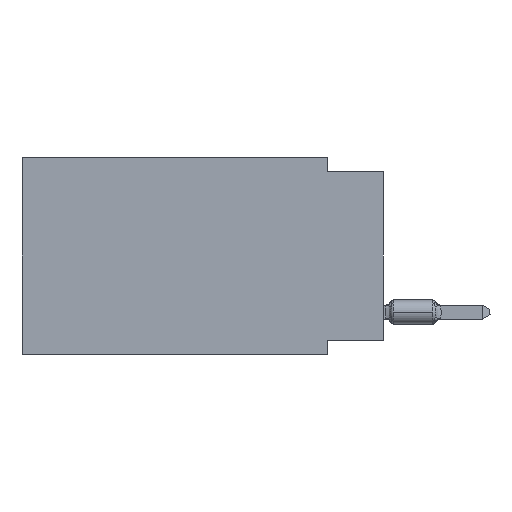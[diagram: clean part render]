
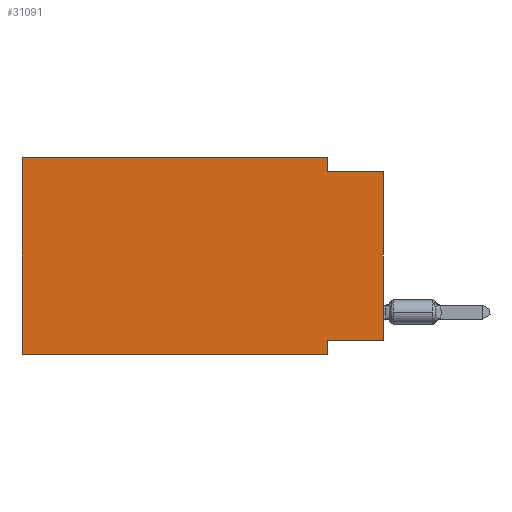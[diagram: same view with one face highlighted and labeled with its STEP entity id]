
A CAD part, left-side view. The second image highlights one B-rep face of the part: STEP entity #31091.
In plain terms, the highlighted planar face has unit normal (-1, 0, 0).
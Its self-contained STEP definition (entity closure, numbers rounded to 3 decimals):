
#676 = VECTOR ( 'NONE', #26741, 1000. ) ;
#1044 = LINE ( 'NONE', #28769, #676 ) ;
#1393 = CARTESIAN_POINT ( 'NONE',  ( 0., 16.383, 0. ) ) ;
#1686 = CARTESIAN_POINT ( 'NONE',  ( 0., 16.383, -8.89 ) ) ;
#1898 = DIRECTION ( 'NONE',  ( 0., 0., -1. ) ) ;
#2497 = VECTOR ( 'NONE', #14791, 1000. ) ;
#2644 = EDGE_CURVE ( 'NONE', #17734, #23725, #25073, .T. ) ;
#3044 = ORIENTED_EDGE ( 'NONE', *, *, #18412, .F. ) ;
#3313 = VERTEX_POINT ( 'NONE', #30371 ) ;
#4046 = ORIENTED_EDGE ( 'NONE', *, *, #2644, .F. ) ;
#4210 = LINE ( 'NONE', #1686, #9690 ) ;
#4249 = VERTEX_POINT ( 'NONE', #11958 ) ;
#4305 = ORIENTED_EDGE ( 'NONE', *, *, #30564, .F. ) ;
#4411 = PLANE ( 'NONE',  #13729 ) ;
#4477 = CARTESIAN_POINT ( 'NONE',  ( 0., 2.54, -8.255 ) ) ;
#4632 = EDGE_CURVE ( 'NONE', #14432, #17476, #32420, .T. ) ;
#4674 = CARTESIAN_POINT ( 'NONE',  ( 0., 2.54, -0.635 ) ) ;
#6158 = CARTESIAN_POINT ( 'NONE',  ( 0., 16.383, 0. ) ) ;
#6249 = VECTOR ( 'NONE', #14885, 1000. ) ;
#6535 = CARTESIAN_POINT ( 'NONE',  ( 0., 16.383, 0. ) ) ;
#6783 = EDGE_CURVE ( 'NONE', #3313, #19375, #8744, .T. ) ;
#6998 = LINE ( 'NONE', #30048, #30743 ) ;
#7349 = DIRECTION ( 'NONE',  ( 0., 0., 1. ) ) ;
#8744 = LINE ( 'NONE', #32408, #9843 ) ;
#9025 = VERTEX_POINT ( 'NONE', #4477 ) ;
#9569 = CARTESIAN_POINT ( 'NONE',  ( 0., 0., -0.635 ) ) ;
#9690 = VECTOR ( 'NONE', #32082, 1000. ) ;
#9843 = VECTOR ( 'NONE', #7349, 1000. ) ;
#9968 = CARTESIAN_POINT ( 'NONE',  ( 0., 2.54, 0. ) ) ;
#11938 = ORIENTED_EDGE ( 'NONE', *, *, #29791, .F. ) ;
#11958 = CARTESIAN_POINT ( 'NONE',  ( 0., 2.54, -8.89 ) ) ;
#12544 = DIRECTION ( 'NONE',  ( 0., 0., -1. ) ) ;
#12728 = ORIENTED_EDGE ( 'NONE', *, *, #4632, .F. ) ;
#12847 = EDGE_CURVE ( 'NONE', #14432, #4249, #4210, .T. ) ;
#12972 = VECTOR ( 'NONE', #14708, 1000. ) ;
#13729 = AXIS2_PLACEMENT_3D ( 'NONE', #1393, #14586, #1898 ) ;
#13777 = EDGE_CURVE ( 'NONE', #23725, #19375, #1044, .T. ) ;
#14094 = FACE_OUTER_BOUND ( 'NONE', #30546, .T. ) ;
#14432 = VERTEX_POINT ( 'NONE', #20504 ) ;
#14586 = DIRECTION ( 'NONE',  ( 1., 0., 0. ) ) ;
#14708 = DIRECTION ( 'NONE',  ( 0., -1., 0. ) ) ;
#14791 = DIRECTION ( 'NONE',  ( 0., 1., 0. ) ) ;
#14885 = DIRECTION ( 'NONE',  ( 0., 0., 1. ) ) ;
#14891 = CARTESIAN_POINT ( 'NONE',  ( 0., 2.54, 0. ) ) ;
#17476 = VERTEX_POINT ( 'NONE', #6158 ) ;
#17734 = VERTEX_POINT ( 'NONE', #9968 ) ;
#18412 = EDGE_CURVE ( 'NONE', #17476, #17734, #19736, .T. ) ;
#19130 = ORIENTED_EDGE ( 'NONE', *, *, #6783, .T. ) ;
#19375 = VERTEX_POINT ( 'NONE', #9569 ) ;
#19736 = LINE ( 'NONE', #6535, #12972 ) ;
#19961 = LINE ( 'NONE', #24483, #2497 ) ;
#20504 = CARTESIAN_POINT ( 'NONE',  ( 0., 16.383, -8.89 ) ) ;
#23725 = VERTEX_POINT ( 'NONE', #4674 ) ;
#24483 = CARTESIAN_POINT ( 'NONE',  ( 0., 0., -8.255 ) ) ;
#24695 = DIRECTION ( 'NONE',  ( 0., 0., -1. ) ) ;
#25073 = LINE ( 'NONE', #14891, #28007 ) ;
#26741 = DIRECTION ( 'NONE',  ( 0., -1., 0. ) ) ;
#27108 = ORIENTED_EDGE ( 'NONE', *, *, #12847, .T. ) ;
#27401 = CARTESIAN_POINT ( 'NONE',  ( 0., 16.383, 0. ) ) ;
#28007 = VECTOR ( 'NONE', #12544, 1000. ) ;
#28404 = ORIENTED_EDGE ( 'NONE', *, *, #13777, .F. ) ;
#28769 = CARTESIAN_POINT ( 'NONE',  ( 0., 0., -0.635 ) ) ;
#29791 = EDGE_CURVE ( 'NONE', #9025, #4249, #6998, .T. ) ;
#30048 = CARTESIAN_POINT ( 'NONE',  ( 0., 2.54, -8.89 ) ) ;
#30371 = CARTESIAN_POINT ( 'NONE',  ( 0., 0., -8.255 ) ) ;
#30546 = EDGE_LOOP ( 'NONE', ( #19130, #28404, #4046, #3044, #12728, #27108, #11938, #4305 ) ) ;
#30564 = EDGE_CURVE ( 'NONE', #3313, #9025, #19961, .T. ) ;
#30743 = VECTOR ( 'NONE', #24695, 1000. ) ;
#31091 = ADVANCED_FACE ( 'NONE', ( #14094 ), #4411, .F. ) ;
#32082 = DIRECTION ( 'NONE',  ( 0., -1., 0. ) ) ;
#32408 = CARTESIAN_POINT ( 'NONE',  ( 0., 0., 0. ) ) ;
#32420 = LINE ( 'NONE', #27401, #6249 ) ;
